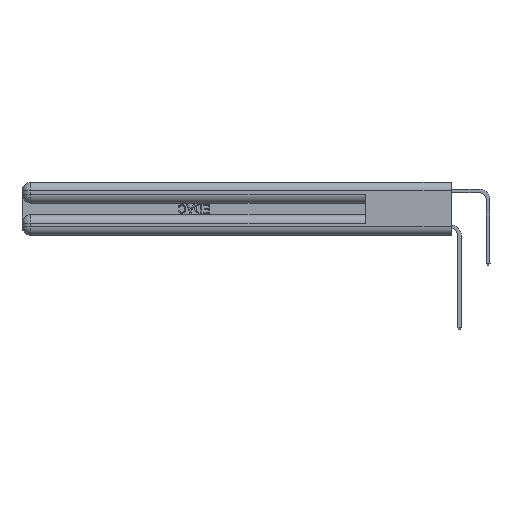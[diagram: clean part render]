
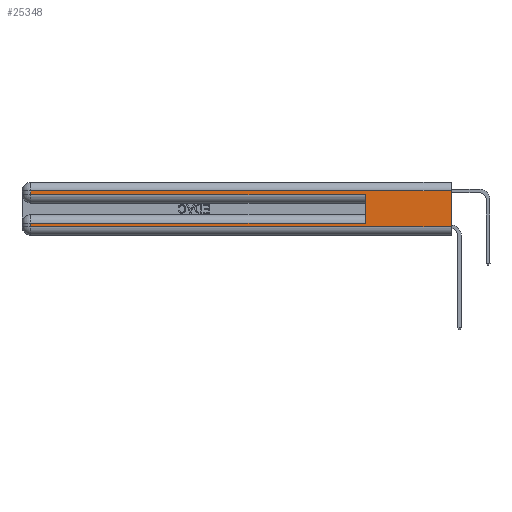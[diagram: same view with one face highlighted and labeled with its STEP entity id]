
A CAD part, left-side view. The second image highlights one B-rep face of the part: STEP entity #25348.
In plain terms, the highlighted planar face has unit normal (-1, 0, 0).
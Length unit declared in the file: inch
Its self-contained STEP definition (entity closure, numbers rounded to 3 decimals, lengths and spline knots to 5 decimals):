
#267 = AXIS2_PLACEMENT_3D ( 'NONE', #5317, #27316, #27014 ) ;
#1085 = EDGE_CURVE ( 'NONE', #17901, #2556, #23962, .T. ) ;
#2018 = CARTESIAN_POINT ( 'NONE',  ( 0., 0.6, 0.085 ) ) ;
#2254 = LINE ( 'NONE', #12052, #14960 ) ;
#2525 = ORIENTED_EDGE ( 'NONE', *, *, #20422, .T. ) ;
#2556 = VERTEX_POINT ( 'NONE', #22494 ) ;
#2710 = DIRECTION ( 'NONE',  ( 0., 0., -1. ) ) ;
#3440 = EDGE_CURVE ( 'NONE', #2556, #11796, #19041, .T. ) ;
#3779 = DIRECTION ( 'NONE',  ( 0., 0., 1. ) ) ;
#4418 = VECTOR ( 'NONE', #2710, 39.37008 ) ;
#4825 = EDGE_LOOP ( 'NONE', ( #30773, #19729, #4849, #7873, #8270, #13755, #2525, #25638 ) ) ;
#4849 = ORIENTED_EDGE ( 'NONE', *, *, #1085, .T. ) ;
#5225 = CARTESIAN_POINT ( 'NONE',  ( 0., 0.6, 0.285 ) ) ;
#5317 = CARTESIAN_POINT ( 'NONE',  ( 0., 0., 0.37 ) ) ;
#6803 = EDGE_CURVE ( 'NONE', #20765, #17901, #2254, .T. ) ;
#6960 = VECTOR ( 'NONE', #11497, 39.37008 ) ;
#7420 = PLANE ( 'NONE',  #267 ) ;
#7523 = VECTOR ( 'NONE', #16265, 39.37008 ) ;
#7873 = ORIENTED_EDGE ( 'NONE', *, *, #3440, .T. ) ;
#8270 = ORIENTED_EDGE ( 'NONE', *, *, #14591, .F. ) ;
#9360 = CARTESIAN_POINT ( 'NONE',  ( 0., 2.94, 0.085 ) ) ;
#9376 = VECTOR ( 'NONE', #28912, 39.37008 ) ;
#9545 = VERTEX_POINT ( 'NONE', #24364 ) ;
#9790 = CARTESIAN_POINT ( 'NONE',  ( 0., 2.94, 0.37 ) ) ;
#9922 = CARTESIAN_POINT ( 'NONE',  ( 0., 0., 0.37 ) ) ;
#11497 = DIRECTION ( 'NONE',  ( 0., -1., 0. ) ) ;
#11796 = VERTEX_POINT ( 'NONE', #5225 ) ;
#12052 = CARTESIAN_POINT ( 'NONE',  ( 0., 0., 0.31 ) ) ;
#12772 = DIRECTION ( 'NONE',  ( 0., 1., 0. ) ) ;
#12933 = LINE ( 'NONE', #25784, #15089 ) ;
#13032 = EDGE_CURVE ( 'NONE', #16921, #18605, #22415, .T. ) ;
#13755 = ORIENTED_EDGE ( 'NONE', *, *, #13032, .T. ) ;
#14591 = EDGE_CURVE ( 'NONE', #16921, #11796, #12933, .T. ) ;
#14615 = DIRECTION ( 'NONE',  ( 0., 1., 0. ) ) ;
#14960 = VECTOR ( 'NONE', #14615, 39.37008 ) ;
#15089 = VECTOR ( 'NONE', #3779, 39.37008 ) ;
#15184 = CARTESIAN_POINT ( 'NONE',  ( 0., 0., 0.31 ) ) ;
#15222 = CARTESIAN_POINT ( 'NONE',  ( 0., 2.94, 0.31 ) ) ;
#15649 = CARTESIAN_POINT ( 'NONE',  ( 0., 0., 0.06 ) ) ;
#16265 = DIRECTION ( 'NONE',  ( 0., 0., -1. ) ) ;
#16727 = CARTESIAN_POINT ( 'NONE',  ( 0., 2.94, 0.37 ) ) ;
#16921 = VERTEX_POINT ( 'NONE', #2018 ) ;
#17368 = FACE_OUTER_BOUND ( 'NONE', #4825, .T. ) ;
#17901 = VERTEX_POINT ( 'NONE', #15222 ) ;
#18062 = LINE ( 'NONE', #15649, #24208 ) ;
#18605 = VERTEX_POINT ( 'NONE', #9360 ) ;
#19041 = LINE ( 'NONE', #23706, #6960 ) ;
#19729 = ORIENTED_EDGE ( 'NONE', *, *, #6803, .T. ) ;
#19755 = LINE ( 'NONE', #9790, #9376 ) ;
#20422 = EDGE_CURVE ( 'NONE', #18605, #9545, #19755, .T. ) ;
#20765 = VERTEX_POINT ( 'NONE', #15184 ) ;
#21079 = EDGE_CURVE ( 'NONE', #9545, #30952, #18062, .T. ) ;
#22415 = LINE ( 'NONE', #27078, #31470 ) ;
#22494 = CARTESIAN_POINT ( 'NONE',  ( 0., 2.94, 0.285 ) ) ;
#23706 = CARTESIAN_POINT ( 'NONE',  ( 0., 0., 0.285 ) ) ;
#23962 = LINE ( 'NONE', #16727, #7523 ) ;
#24208 = VECTOR ( 'NONE', #27848, 39.37008 ) ;
#24364 = CARTESIAN_POINT ( 'NONE',  ( 0., 2.94, 0.06 ) ) ;
#24418 = CARTESIAN_POINT ( 'NONE',  ( 0., 0., 0.06 ) ) ;
#25348 = ADVANCED_FACE ( 'NONE', ( #17368 ), #7420, .F. ) ;
#25638 = ORIENTED_EDGE ( 'NONE', *, *, #21079, .T. ) ;
#25766 = EDGE_CURVE ( 'NONE', #20765, #30952, #27277, .T. ) ;
#25784 = CARTESIAN_POINT ( 'NONE',  ( 0., 0.6, 0.145 ) ) ;
#27014 = DIRECTION ( 'NONE',  ( 0., 0., -1. ) ) ;
#27078 = CARTESIAN_POINT ( 'NONE',  ( 0., 0., 0.085 ) ) ;
#27277 = LINE ( 'NONE', #9922, #4418 ) ;
#27316 = DIRECTION ( 'NONE',  ( 1., 0., 0. ) ) ;
#27848 = DIRECTION ( 'NONE',  ( 0., -1., 0. ) ) ;
#28912 = DIRECTION ( 'NONE',  ( 0., 0., -1. ) ) ;
#30773 = ORIENTED_EDGE ( 'NONE', *, *, #25766, .F. ) ;
#30952 = VERTEX_POINT ( 'NONE', #24418 ) ;
#31470 = VECTOR ( 'NONE', #12772, 39.37008 ) ;
